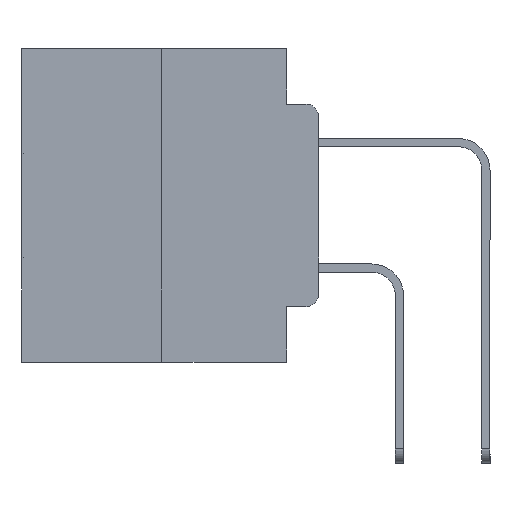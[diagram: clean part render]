
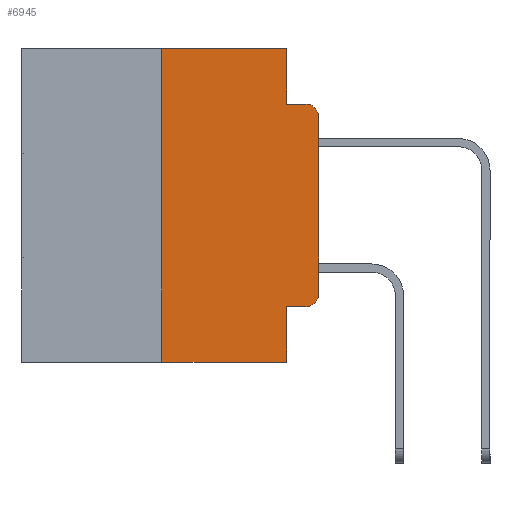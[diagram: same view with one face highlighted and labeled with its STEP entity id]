
A CAD part, left-side view. The second image highlights one B-rep face of the part: STEP entity #6945.
In plain terms, the highlighted planar face has unit normal (-1, 0, 0).
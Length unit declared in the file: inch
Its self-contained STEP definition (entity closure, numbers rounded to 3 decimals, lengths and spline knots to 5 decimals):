
#225 = CIRCLE ( 'NONE', #4014, 0.02 ) ;
#632 = DIRECTION ( 'NONE',  ( 1., 0., 0. ) ) ;
#1094 = CARTESIAN_POINT ( 'NONE',  ( 0., 0.02, -0.4115 ) ) ;
#1212 = CARTESIAN_POINT ( 'NONE',  ( 0., 0.25, -0.5 ) ) ;
#1289 = VECTOR ( 'NONE', #13509, 39.37008 ) ;
#1398 = VECTOR ( 'NONE', #2333, 39.37008 ) ;
#2333 = DIRECTION ( 'NONE',  ( 0., 0., -1. ) ) ;
#2609 = ORIENTED_EDGE ( 'NONE', *, *, #7494, .T. ) ;
#2680 = AXIS2_PLACEMENT_3D ( 'NONE', #3631, #19319, #5885 ) ;
#3097 = VECTOR ( 'NONE', #26845, 39.37008 ) ;
#3631 = CARTESIAN_POINT ( 'NONE',  ( 0., 0.02, -0.1085 ) ) ;
#3935 = VERTEX_POINT ( 'NONE', #26574 ) ;
#4014 = AXIS2_PLACEMENT_3D ( 'NONE', #9295, #24845, #11538 ) ;
#4128 = VERTEX_POINT ( 'NONE', #16329 ) ;
#4593 = CARTESIAN_POINT ( 'NONE',  ( 0., 0., 0. ) ) ;
#4705 = ORIENTED_EDGE ( 'NONE', *, *, #21510, .F. ) ;
#4868 = LINE ( 'NONE', #7805, #16095 ) ;
#5421 = VECTOR ( 'NONE', #18391, 39.37008 ) ;
#5885 = DIRECTION ( 'NONE',  ( 0., 0., -1. ) ) ;
#6097 = ORIENTED_EDGE ( 'NONE', *, *, #26964, .F. ) ;
#6286 = CARTESIAN_POINT ( 'NONE',  ( 0., 0.051, 0. ) ) ;
#6819 = LINE ( 'NONE', #11619, #5421 ) ;
#6945 = ADVANCED_FACE ( 'NONE', ( #9673 ), #14052, .F. ) ;
#7273 = LINE ( 'NONE', #24596, #1289 ) ;
#7494 = EDGE_CURVE ( 'NONE', #18167, #17815, #14851, .T. ) ;
#7541 = ORIENTED_EDGE ( 'NONE', *, *, #12395, .T. ) ;
#7805 = CARTESIAN_POINT ( 'NONE',  ( 0., 0.473, -0.5 ) ) ;
#8999 = EDGE_CURVE ( 'NONE', #17815, #23384, #16549, .T. ) ;
#9069 = CARTESIAN_POINT ( 'NONE',  ( 0., 0.051, -0.0885 ) ) ;
#9143 = DIRECTION ( 'NONE',  ( 0., 0., 1. ) ) ;
#9295 = CARTESIAN_POINT ( 'NONE',  ( 0., 0.02, -0.3915 ) ) ;
#9417 = CARTESIAN_POINT ( 'NONE',  ( 0., 0., -0.1085 ) ) ;
#9673 = FACE_OUTER_BOUND ( 'NONE', #17564, .T. ) ;
#10077 = DIRECTION ( 'NONE',  ( 0., -1., 0. ) ) ;
#10698 = LINE ( 'NONE', #15022, #21827 ) ;
#11317 = VERTEX_POINT ( 'NONE', #1094 ) ;
#11538 = DIRECTION ( 'NONE',  ( 0., 0., -1. ) ) ;
#11619 = CARTESIAN_POINT ( 'NONE',  ( 0., 0.473, 0. ) ) ;
#12395 = EDGE_CURVE ( 'NONE', #11317, #18167, #225, .T. ) ;
#13268 = EDGE_CURVE ( 'NONE', #14006, #11317, #10698, .T. ) ;
#13320 = VERTEX_POINT ( 'NONE', #6286 ) ;
#13509 = DIRECTION ( 'NONE',  ( 0., 0., -1. ) ) ;
#14006 = VERTEX_POINT ( 'NONE', #19673 ) ;
#14052 = PLANE ( 'NONE',  #14112 ) ;
#14112 = AXIS2_PLACEMENT_3D ( 'NONE', #27326, #632, #16321 ) ;
#14851 = LINE ( 'NONE', #4593, #25947 ) ;
#15022 = CARTESIAN_POINT ( 'NONE',  ( 0., 0.051, -0.4115 ) ) ;
#15239 = CARTESIAN_POINT ( 'NONE',  ( 0., 0.25, 0. ) ) ;
#15518 = VECTOR ( 'NONE', #24176, 39.37008 ) ;
#15572 = CARTESIAN_POINT ( 'NONE',  ( 0., 0.051, -0.5 ) ) ;
#15936 = ORIENTED_EDGE ( 'NONE', *, *, #25206, .F. ) ;
#16095 = VECTOR ( 'NONE', #10077, 39.37008 ) ;
#16321 = DIRECTION ( 'NONE',  ( 0., 0., -1. ) ) ;
#16329 = CARTESIAN_POINT ( 'NONE',  ( 0., 0.051, -0.0885 ) ) ;
#16549 = CIRCLE ( 'NONE', #2680, 0.02 ) ;
#17034 = VERTEX_POINT ( 'NONE', #15572 ) ;
#17303 = DIRECTION ( 'NONE',  ( 0., -1., 0. ) ) ;
#17316 = CARTESIAN_POINT ( 'NONE',  ( 0., 0., -0.3915 ) ) ;
#17564 = EDGE_LOOP ( 'NONE', ( #2609, #21156, #27021, #15936, #21832, #4705, #22530, #6097, #18076, #7541 ) ) ;
#17815 = VERTEX_POINT ( 'NONE', #9417 ) ;
#18076 = ORIENTED_EDGE ( 'NONE', *, *, #13268, .T. ) ;
#18167 = VERTEX_POINT ( 'NONE', #17316 ) ;
#18391 = DIRECTION ( 'NONE',  ( 0., -1., 0. ) ) ;
#18886 = EDGE_CURVE ( 'NONE', #4128, #23384, #26796, .T. ) ;
#19286 = LINE ( 'NONE', #26801, #1398 ) ;
#19319 = DIRECTION ( 'NONE',  ( -1., 0., 0. ) ) ;
#19673 = CARTESIAN_POINT ( 'NONE',  ( 0., 0.051, -0.4115 ) ) ;
#20770 = EDGE_CURVE ( 'NONE', #3935, #13320, #6819, .T. ) ;
#21156 = ORIENTED_EDGE ( 'NONE', *, *, #8999, .T. ) ;
#21457 = LINE ( 'NONE', #15239, #15518 ) ;
#21510 = EDGE_CURVE ( 'NONE', #23802, #3935, #21457, .T. ) ;
#21827 = VECTOR ( 'NONE', #17303, 39.37008 ) ;
#21832 = ORIENTED_EDGE ( 'NONE', *, *, #20770, .F. ) ;
#22530 = ORIENTED_EDGE ( 'NONE', *, *, #25983, .T. ) ;
#23384 = VERTEX_POINT ( 'NONE', #28682 ) ;
#23802 = VERTEX_POINT ( 'NONE', #1212 ) ;
#24176 = DIRECTION ( 'NONE',  ( 0., 0., 1. ) ) ;
#24596 = CARTESIAN_POINT ( 'NONE',  ( 0., 0.051, 0. ) ) ;
#24845 = DIRECTION ( 'NONE',  ( -1., 0., 0. ) ) ;
#25206 = EDGE_CURVE ( 'NONE', #13320, #4128, #19286, .T. ) ;
#25947 = VECTOR ( 'NONE', #9143, 39.37008 ) ;
#25983 = EDGE_CURVE ( 'NONE', #23802, #17034, #4868, .T. ) ;
#26574 = CARTESIAN_POINT ( 'NONE',  ( 0., 0.25, 0. ) ) ;
#26796 = LINE ( 'NONE', #9069, #3097 ) ;
#26801 = CARTESIAN_POINT ( 'NONE',  ( 0., 0.051, 0. ) ) ;
#26845 = DIRECTION ( 'NONE',  ( 0., -1., 0. ) ) ;
#26964 = EDGE_CURVE ( 'NONE', #14006, #17034, #7273, .T. ) ;
#27021 = ORIENTED_EDGE ( 'NONE', *, *, #18886, .F. ) ;
#27326 = CARTESIAN_POINT ( 'NONE',  ( 0., 0.473, 0. ) ) ;
#28682 = CARTESIAN_POINT ( 'NONE',  ( 0., 0.02, -0.0885 ) ) ;
